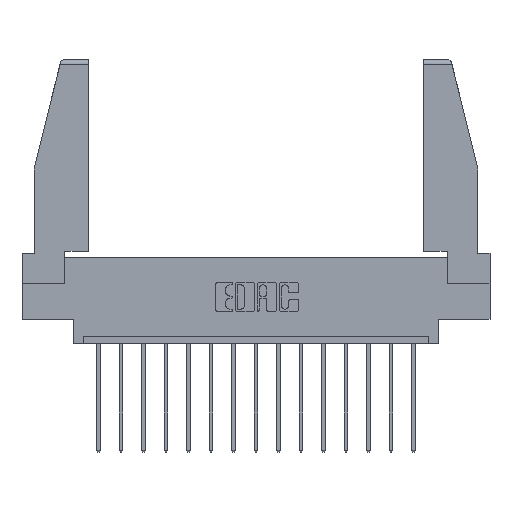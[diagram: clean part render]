
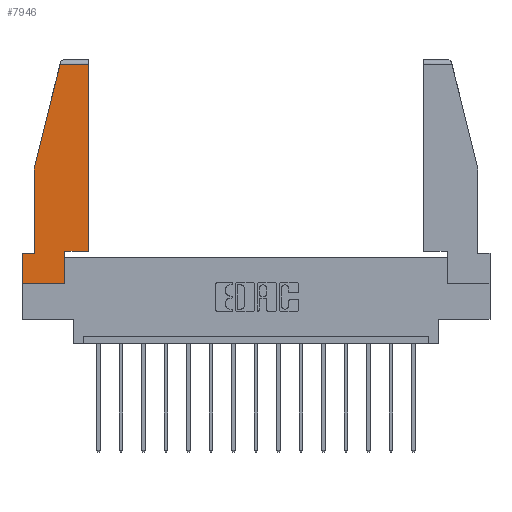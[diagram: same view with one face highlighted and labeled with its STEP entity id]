
A CAD part, top view. The second image highlights one B-rep face of the part: STEP entity #7946.
In plain terms, the highlighted planar face has unit normal (0, 0, 1).
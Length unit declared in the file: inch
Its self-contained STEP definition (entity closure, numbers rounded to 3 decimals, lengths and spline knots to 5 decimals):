
#225 = CARTESIAN_POINT ( 'NONE',  ( 0., 0.21, 0. ) ) ;
#242 = VERTEX_POINT ( 'NONE', #1253 ) ;
#254 = ORIENTED_EDGE ( 'NONE', *, *, #13701, .T. ) ;
#868 = LINE ( 'NONE', #11306, #7165 ) ;
#877 = DIRECTION ( 'NONE',  ( 0., 1., 0. ) ) ;
#1253 = CARTESIAN_POINT ( 'NONE',  ( 0.086, 0.21, 0. ) ) ;
#1474 = CARTESIAN_POINT ( 'NONE',  ( 0.271, 1.55, 0. ) ) ;
#1588 = CARTESIAN_POINT ( 'NONE',  ( 0.297, 0., 0. ) ) ;
#1873 = VERTEX_POINT ( 'NONE', #1588 ) ;
#2236 = ORIENTED_EDGE ( 'NONE', *, *, #9212, .T. ) ;
#2266 = CARTESIAN_POINT ( 'NONE',  ( 0., 0., 0. ) ) ;
#2302 = ORIENTED_EDGE ( 'NONE', *, *, #12358, .T. ) ;
#2377 = LINE ( 'NONE', #9817, #12611 ) ;
#2384 = VERTEX_POINT ( 'NONE', #7883 ) ;
#2444 = ORIENTED_EDGE ( 'NONE', *, *, #13883, .T. ) ;
#2786 = ORIENTED_EDGE ( 'NONE', *, *, #7674, .T. ) ;
#2937 = VECTOR ( 'NONE', #6589, 39.37008 ) ;
#3028 = DIRECTION ( 'NONE',  ( 1., 0., 0. ) ) ;
#3124 = LINE ( 'NONE', #225, #5018 ) ;
#3716 = DIRECTION ( 'NONE',  ( 0., 0., 1. ) ) ;
#4046 = VERTEX_POINT ( 'NONE', #14750 ) ;
#5018 = VECTOR ( 'NONE', #13667, 39.37008 ) ;
#5697 = CARTESIAN_POINT ( 'NONE',  ( 0.2636, 1.52, 0. ) ) ;
#6350 = ORIENTED_EDGE ( 'NONE', *, *, #13462, .T. ) ;
#6389 = VERTEX_POINT ( 'NONE', #10209 ) ;
#6478 = DIRECTION ( 'NONE',  ( 1., 0., 0. ) ) ;
#6589 = DIRECTION ( 'NONE',  ( 1., 0., 0. ) ) ;
#7165 = VECTOR ( 'NONE', #16651, 39.37008 ) ;
#7287 = VECTOR ( 'NONE', #877, 39.37008 ) ;
#7637 = VECTOR ( 'NONE', #15793, 39.37008 ) ;
#7674 = EDGE_CURVE ( 'NONE', #9513, #9205, #14690, .T. ) ;
#7883 = CARTESIAN_POINT ( 'NONE',  ( 0.297, 0.223, 0. ) ) ;
#7946 = ADVANCED_FACE ( 'NONE', ( #13437 ), #15608, .T. ) ;
#7959 = VERTEX_POINT ( 'NONE', #14321 ) ;
#8005 = DIRECTION ( 'NONE',  ( -0.239, -0.971, 0. ) ) ;
#8107 = CARTESIAN_POINT ( 'NONE',  ( 0.086, 0.8, 0. ) ) ;
#8373 = LINE ( 'NONE', #9169, #2937 ) ;
#8678 = LINE ( 'NONE', #14378, #7637 ) ;
#9169 = CARTESIAN_POINT ( 'NONE',  ( 0.297, 0.223, 0. ) ) ;
#9205 = VERTEX_POINT ( 'NONE', #9662 ) ;
#9212 = EDGE_CURVE ( 'NONE', #242, #6389, #3124, .T. ) ;
#9513 = VERTEX_POINT ( 'NONE', #5697 ) ;
#9662 = CARTESIAN_POINT ( 'NONE',  ( 0.086, 0.8, 0. ) ) ;
#9817 = CARTESIAN_POINT ( 'NONE',  ( 0., 0., 0. ) ) ;
#10017 = LINE ( 'NONE', #14599, #11463 ) ;
#10209 = CARTESIAN_POINT ( 'NONE',  ( 0., 0.21, 0. ) ) ;
#10239 = VECTOR ( 'NONE', #12194, 39.37008 ) ;
#10669 = DIRECTION ( 'NONE',  ( 0., -1., 0. ) ) ;
#11306 = CARTESIAN_POINT ( 'NONE',  ( 0.297, 0., 0. ) ) ;
#11463 = VECTOR ( 'NONE', #10669, 39.37008 ) ;
#11551 = VERTEX_POINT ( 'NONE', #16862 ) ;
#12194 = DIRECTION ( 'NONE',  ( 0., -1., 0. ) ) ;
#12292 = LINE ( 'NONE', #16890, #7287 ) ;
#12358 = EDGE_CURVE ( 'NONE', #4046, #1873, #2377, .T. ) ;
#12611 = VECTOR ( 'NONE', #3028, 39.37008 ) ;
#13148 = EDGE_LOOP ( 'NONE', ( #14253, #15518, #2786, #2444, #2236, #13536, #2302, #6350, #254 ) ) ;
#13166 = LINE ( 'NONE', #8107, #10239 ) ;
#13437 = FACE_OUTER_BOUND ( 'NONE', #13148, .T. ) ;
#13462 = EDGE_CURVE ( 'NONE', #1873, #2384, #868, .T. ) ;
#13536 = ORIENTED_EDGE ( 'NONE', *, *, #14469, .T. ) ;
#13667 = DIRECTION ( 'NONE',  ( -1., 0., 0. ) ) ;
#13701 = EDGE_CURVE ( 'NONE', #2384, #7959, #8373, .T. ) ;
#13883 = EDGE_CURVE ( 'NONE', #9205, #242, #13166, .T. ) ;
#14253 = ORIENTED_EDGE ( 'NONE', *, *, #15396, .T. ) ;
#14321 = CARTESIAN_POINT ( 'NONE',  ( 0.461, 0.223, 0. ) ) ;
#14378 = CARTESIAN_POINT ( 'NONE',  ( 0., 1.52, 0. ) ) ;
#14469 = EDGE_CURVE ( 'NONE', #6389, #4046, #10017, .T. ) ;
#14599 = CARTESIAN_POINT ( 'NONE',  ( 0., 0.21, 0. ) ) ;
#14690 = LINE ( 'NONE', #1474, #16565 ) ;
#14750 = CARTESIAN_POINT ( 'NONE',  ( 0., 0., 0. ) ) ;
#15396 = EDGE_CURVE ( 'NONE', #7959, #11551, #12292, .T. ) ;
#15518 = ORIENTED_EDGE ( 'NONE', *, *, #15748, .T. ) ;
#15608 = PLANE ( 'NONE',  #16558 ) ;
#15748 = EDGE_CURVE ( 'NONE', #11551, #9513, #8678, .T. ) ;
#15793 = DIRECTION ( 'NONE',  ( -1., 0., 0. ) ) ;
#16558 = AXIS2_PLACEMENT_3D ( 'NONE', #2266, #3716, #6478 ) ;
#16565 = VECTOR ( 'NONE', #8005, 39.37008 ) ;
#16651 = DIRECTION ( 'NONE',  ( 0., 1., 0. ) ) ;
#16862 = CARTESIAN_POINT ( 'NONE',  ( 0.461, 1.52, 0. ) ) ;
#16890 = CARTESIAN_POINT ( 'NONE',  ( 0.461, 0.223, 0. ) ) ;
